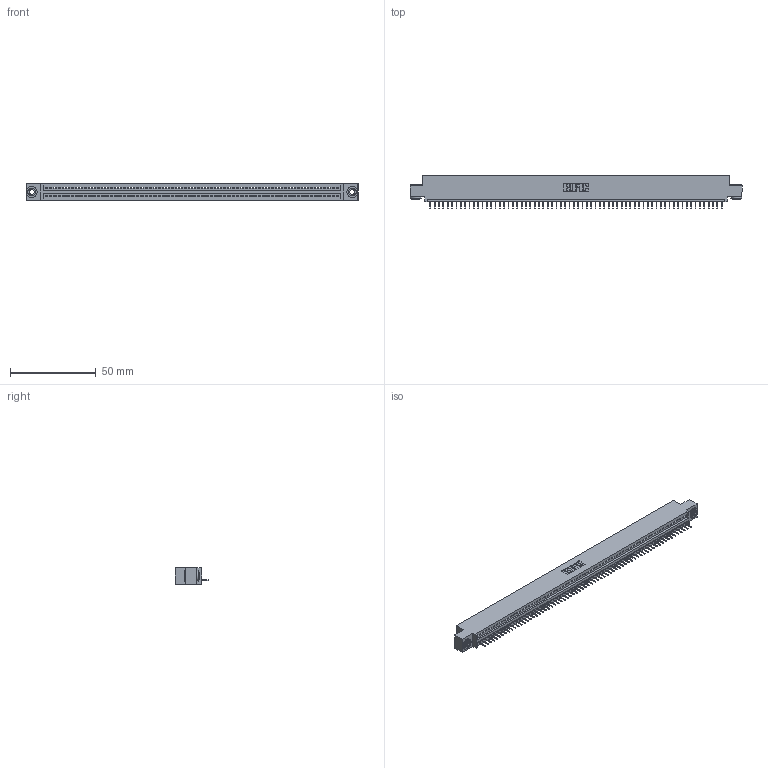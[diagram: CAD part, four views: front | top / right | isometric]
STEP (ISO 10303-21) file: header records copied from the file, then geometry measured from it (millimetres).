
FILE_DESCRIPTION (( 'STEP AP203' ), '1' );
FILE_NAME ('395-068-524-403.STEP', '2019-10-25T16:22:29', ( '' ), ( '' ), 'SwSTEP 2.0', 'SolidWorks 2016', '' );
FILE_SCHEMA (( 'CONFIG_CONTROL_DESIGN' ));
Length unit declared in the file: inch
Products named in the file (4): 345 Part_0.110 Offset - 0.156 Dia-TH; 345-292-001_345-293-124; 395-068-524-403; 345-250-002_345-250-002-102
Assembly tree (71 placements, depth 2):
  395-068-524-403
    345 Part_0.110 Offset - 0.156 Dia-TH
    345-292-001_345-293-124  x68
    345-250-002_345-250-002-102  x2
Bounding box: 193.93 x 19.35 x 9.4 mm (x, y, z)
Volume: 18310 mm3; surface area: 24123.1 mm2
Topology: 71 solids, 71 shells, 4384 faces, 12669 edges, 8170 vertices
Faces by surface type: plane 3222, cylinder 1154, cone 8
Entity records: 48534 total; most frequent: CARTESIAN_POINT 8383, ORIENTED_EDGE 8378, DIRECTION 7315, EDGE_CURVE 4189, VECTOR 3765, LINE 3765, VERTEX_POINT 2786, AXIS2_PLACEMENT_3D 1775
